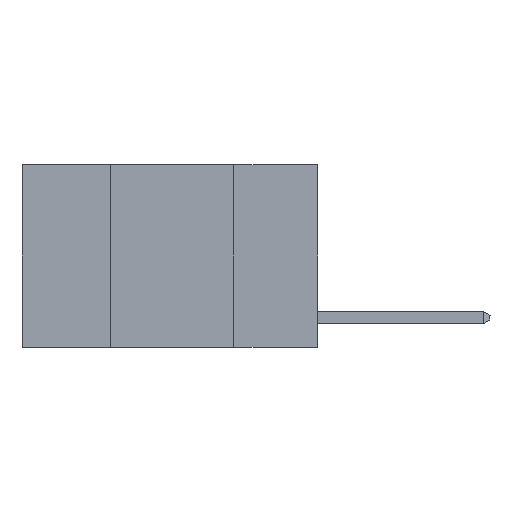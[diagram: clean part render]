
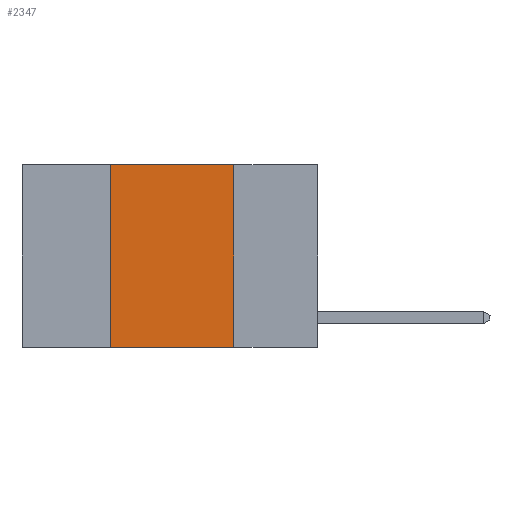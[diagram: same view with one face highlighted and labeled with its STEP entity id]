
A CAD part, left-side view. The second image highlights one B-rep face of the part: STEP entity #2347.
In plain terms, the highlighted planar face has unit normal (-1, 0, 0).
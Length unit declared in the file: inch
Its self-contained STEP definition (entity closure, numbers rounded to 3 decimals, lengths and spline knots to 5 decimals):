
#91 = CARTESIAN_POINT ( 'NONE',  ( 0., 0.6, 0. ) ) ;
#445 = EDGE_LOOP ( 'NONE', ( #7960, #9319, #1630, #2583 ) ) ;
#658 = LINE ( 'NONE', #91, #8891 ) ;
#944 = EDGE_CURVE ( 'NONE', #7955, #5266, #3179, .T. ) ;
#976 = CARTESIAN_POINT ( 'NONE',  ( 0., 0.17, 0. ) ) ;
#1630 = ORIENTED_EDGE ( 'NONE', *, *, #7635, .F. ) ;
#2099 = LINE ( 'NONE', #4742, #6189 ) ;
#2347 = ADVANCED_FACE ( 'NONE', ( #5584 ), #8996, .F. ) ;
#2500 = VECTOR ( 'NONE', #6123, 39.37008 ) ;
#2520 = DIRECTION ( 'NONE',  ( 0., 0., 1. ) ) ;
#2583 = ORIENTED_EDGE ( 'NONE', *, *, #5496, .T. ) ;
#2635 = DIRECTION ( 'NONE',  ( 0., 0., -1. ) ) ;
#2833 = VECTOR ( 'NONE', #8537, 39.37008 ) ;
#3179 = LINE ( 'NONE', #976, #2833 ) ;
#4742 = CARTESIAN_POINT ( 'NONE',  ( 0., 0.42, 0. ) ) ;
#5134 = VERTEX_POINT ( 'NONE', #6170 ) ;
#5266 = VERTEX_POINT ( 'NONE', #6427 ) ;
#5496 = EDGE_CURVE ( 'NONE', #5134, #5266, #8348, .T. ) ;
#5500 = CARTESIAN_POINT ( 'NONE',  ( 0., 0.6, 0. ) ) ;
#5578 = AXIS2_PLACEMENT_3D ( 'NONE', #5500, #9306, #2635 ) ;
#5584 = FACE_OUTER_BOUND ( 'NONE', #445, .T. ) ;
#5786 = CARTESIAN_POINT ( 'NONE',  ( 0., 0.42, 0. ) ) ;
#6123 = DIRECTION ( 'NONE',  ( 0., -1., 0. ) ) ;
#6170 = CARTESIAN_POINT ( 'NONE',  ( 0., 0.42, -0.37 ) ) ;
#6189 = VECTOR ( 'NONE', #2520, 39.37008 ) ;
#6427 = CARTESIAN_POINT ( 'NONE',  ( 0., 0.17, -0.37 ) ) ;
#6929 = CARTESIAN_POINT ( 'NONE',  ( 0., 0.6, -0.37 ) ) ;
#7187 = CARTESIAN_POINT ( 'NONE',  ( 0., 0.17, 0. ) ) ;
#7543 = EDGE_CURVE ( 'NONE', #8292, #7955, #658, .T. ) ;
#7635 = EDGE_CURVE ( 'NONE', #5134, #8292, #2099, .T. ) ;
#7955 = VERTEX_POINT ( 'NONE', #7187 ) ;
#7960 = ORIENTED_EDGE ( 'NONE', *, *, #944, .F. ) ;
#8292 = VERTEX_POINT ( 'NONE', #5786 ) ;
#8309 = DIRECTION ( 'NONE',  ( 0., -1., 0. ) ) ;
#8348 = LINE ( 'NONE', #6929, #2500 ) ;
#8537 = DIRECTION ( 'NONE',  ( 0., 0., -1. ) ) ;
#8891 = VECTOR ( 'NONE', #8309, 39.37008 ) ;
#8996 = PLANE ( 'NONE',  #5578 ) ;
#9306 = DIRECTION ( 'NONE',  ( 1., 0., 0. ) ) ;
#9319 = ORIENTED_EDGE ( 'NONE', *, *, #7543, .F. ) ;
